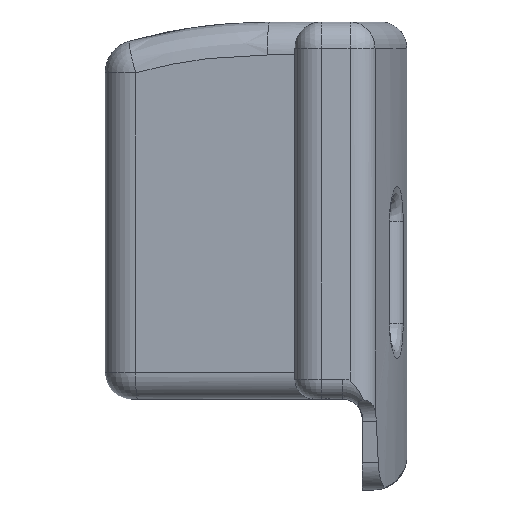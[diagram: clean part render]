
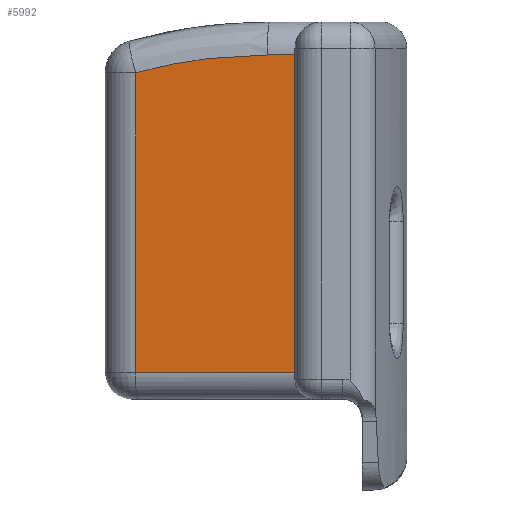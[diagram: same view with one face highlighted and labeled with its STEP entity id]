
A CAD part, left-side view. The second image highlights one B-rep face of the part: STEP entity #5992.
In plain terms, the highlighted planar face has unit normal (-0.997, 0.075, 0).
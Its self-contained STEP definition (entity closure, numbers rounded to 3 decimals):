
#81 = AXIS2_PLACEMENT_3D ( 'NONE', #7341, #6042, #1817 ) ;
#185 = CARTESIAN_POINT ( 'NONE',  ( 33.949, 71.388, 90.508 ) ) ;
#222 = CARTESIAN_POINT ( 'NONE',  ( 32.135, 47.214, 90.508 ) ) ;
#226 = CARTESIAN_POINT ( 'NONE',  ( 32.45, 51.408, 85.508 ) ) ;
#427 = CARTESIAN_POINT ( 'NONE',  ( 33.949, 71.388, 37.308 ) ) ;
#449 = CARTESIAN_POINT ( 'NONE',  ( 33.46, 64.871, 84.599 ) ) ;
#638 = EDGE_CURVE ( 'NONE', #3334, #1524, #906, .T. ) ;
#875 = VECTOR ( 'NONE', #1620, 1000. ) ;
#906 =( BOUNDED_CURVE ( )  B_SPLINE_CURVE ( 3, ( #1026, #2462, #449, #2340 ),
 .UNSPECIFIED., .F., .F. ) 
 B_SPLINE_CURVE_WITH_KNOTS ( ( 4, 4 ),
 ( 1.571, 1.84 ),
 .UNSPECIFIED. ) 
 CURVE ( )  GEOMETRIC_REPRESENTATION_ITEM ( )  RATIONAL_B_SPLINE_CURVE ( ( 1., 0.994, 0.994, 1. ) ) 
 REPRESENTATION_ITEM ( '' )  );
#1026 = CARTESIAN_POINT ( 'NONE',  ( 32.45, 51.408, 85.508 ) ) ;
#1208 = CARTESIAN_POINT ( 'NONE',  ( 32.135, 47.214, 90.508 ) ) ;
#1524 = VERTEX_POINT ( 'NONE', #3456 ) ;
#1547 = CARTESIAN_POINT ( 'NONE',  ( 33.949, 71.388, 85.508 ) ) ;
#1620 = DIRECTION ( 'NONE',  ( 0.075, 0.997, 0. ) ) ;
#1817 = DIRECTION ( 'NONE',  ( 0.075, 0.997, 0. ) ) ;
#2340 = CARTESIAN_POINT ( 'NONE',  ( 33.949, 71.388, 82.798 ) ) ;
#2462 = CARTESIAN_POINT ( 'NONE',  ( 32.957, 58.17, 85.508 ) ) ;
#2469 = EDGE_LOOP ( 'NONE', ( #2648, #4471, #2814, #7021, #5824, #7988 ) ) ;
#2471 = DIRECTION ( 'NONE',  ( -0.075, -0.997, 0. ) ) ;
#2569 = VECTOR ( 'NONE', #2471, 1000. ) ;
#2648 = ORIENTED_EDGE ( 'NONE', *, *, #6049, .F. ) ;
#2661 = LINE ( 'NONE', #185, #2787 ) ;
#2786 = VERTEX_POINT ( 'NONE', #7047 ) ;
#2787 = VECTOR ( 'NONE', #6439, 1000. ) ;
#2814 = ORIENTED_EDGE ( 'NONE', *, *, #638, .T. ) ;
#2883 = DIRECTION ( 'NONE',  ( 0., 0., -1. ) ) ;
#2992 = EDGE_CURVE ( 'NONE', #1524, #7140, #2661, .T. ) ;
#3055 = DIRECTION ( 'NONE',  ( 0., 0., -1. ) ) ;
#3334 = VERTEX_POINT ( 'NONE', #226 ) ;
#3456 = CARTESIAN_POINT ( 'NONE',  ( 33.949, 71.388, 82.798 ) ) ;
#3593 = PLANE ( 'NONE',  #81 ) ;
#3603 = VERTEX_POINT ( 'NONE', #4056 ) ;
#4022 = VECTOR ( 'NONE', #3055, 1000. ) ;
#4056 = CARTESIAN_POINT ( 'NONE',  ( 32.135, 47.214, 83.508 ) ) ;
#4347 = EDGE_CURVE ( 'NONE', #3603, #2786, #4446, .T. ) ;
#4383 = VERTEX_POINT ( 'NONE', #5207 ) ;
#4446 = LINE ( 'NONE', #222, #4924 ) ;
#4471 = ORIENTED_EDGE ( 'NONE', *, *, #7970, .T. ) ;
#4924 = VECTOR ( 'NONE', #2883, 1000. ) ;
#5207 = CARTESIAN_POINT ( 'NONE',  ( 32.135, 47.214, 85.508 ) ) ;
#5824 = ORIENTED_EDGE ( 'NONE', *, *, #6755, .T. ) ;
#5992 = ADVANCED_FACE ( 'NONE', ( #7458 ), #3593, .F. ) ;
#6042 = DIRECTION ( 'NONE',  ( 0.997, -0.075, 0. ) ) ;
#6049 = EDGE_CURVE ( 'NONE', #4383, #3603, #6753, .T. ) ;
#6126 = LINE ( 'NONE', #6747, #2569 ) ;
#6439 = DIRECTION ( 'NONE',  ( 0., 0., -1. ) ) ;
#6747 = CARTESIAN_POINT ( 'NONE',  ( 32.135, 47.214, 37.308 ) ) ;
#6753 = LINE ( 'NONE', #1208, #4022 ) ;
#6755 = EDGE_CURVE ( 'NONE', #7140, #2786, #6126, .T. ) ;
#7021 = ORIENTED_EDGE ( 'NONE', *, *, #2992, .T. ) ;
#7047 = CARTESIAN_POINT ( 'NONE',  ( 32.135, 47.214, 37.308 ) ) ;
#7140 = VERTEX_POINT ( 'NONE', #427 ) ;
#7148 = LINE ( 'NONE', #1547, #875 ) ;
#7341 = CARTESIAN_POINT ( 'NONE',  ( 33.949, 71.388, 90.508 ) ) ;
#7458 = FACE_OUTER_BOUND ( 'NONE', #2469, .T. ) ;
#7970 = EDGE_CURVE ( 'NONE', #4383, #3334, #7148, .T. ) ;
#7988 = ORIENTED_EDGE ( 'NONE', *, *, #4347, .F. ) ;
